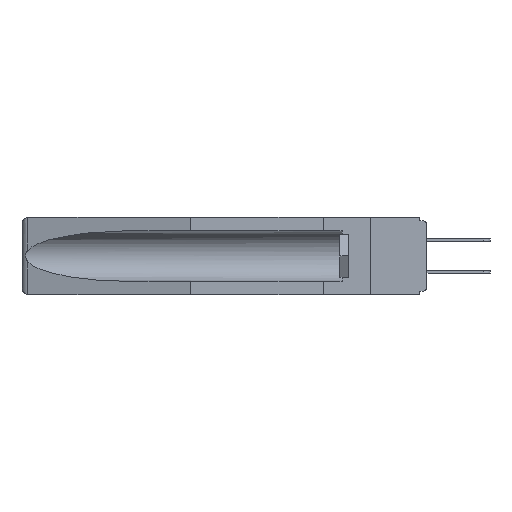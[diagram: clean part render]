
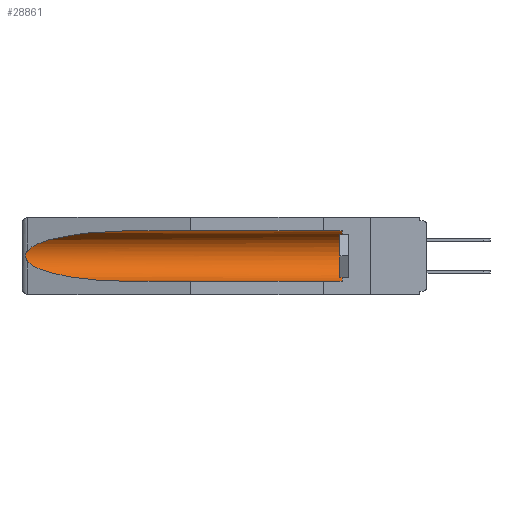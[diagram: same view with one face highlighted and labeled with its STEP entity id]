
A CAD part, left-side view. The second image highlights one B-rep face of the part: STEP entity #28861.
In plain terms, the highlighted cylindrical face has radius 2.857 mm (diameter 5.715 mm), a partial arc.
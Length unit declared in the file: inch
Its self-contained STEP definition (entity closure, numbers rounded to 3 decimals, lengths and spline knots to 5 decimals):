
#304 = CARTESIAN_POINT ( 'NONE',  ( 0.155, 1.07973, -0.284 ) ) ;
#995 = CARTESIAN_POINT ( 'NONE',  ( 0.26537, 1.52718, -0.19328 ) ) ;
#2540 = CARTESIAN_POINT ( 'NONE',  ( 0.26537, 1.52718, -0.19328 ) ) ;
#2613 = EDGE_CURVE ( 'NONE', #5798, #22632, #31333, .T. ) ;
#2690 = CARTESIAN_POINT ( 'NONE',  ( 0.155, -0.30754, -0.284 ) ) ;
#3827 = DIRECTION ( 'NONE',  ( 0., 1., 0. ) ) ;
#4141 = CARTESIAN_POINT ( 'NONE',  ( 0.155, 0.126, -0.284 ) ) ;
#4166 = EDGE_CURVE ( 'NONE', #13967, #22632, #28898, .T. ) ;
#4778 = CARTESIAN_POINT ( 'NONE',  ( 0.26654, 1.53092, -0.15636 ) ) ;
#5798 = VERTEX_POINT ( 'NONE', #4141 ) ;
#6088 = ORIENTED_EDGE ( 'NONE', *, *, #4166, .T. ) ;
#6415 = CYLINDRICAL_SURFACE ( 'NONE', #23253, 0.1125 ) ;
#6547 = CIRCLE ( 'NONE', #26962, 0.1125 ) ;
#7343 = CARTESIAN_POINT ( 'NONE',  ( 0.21114, 1.30732, -0.059 ) ) ;
#7671 = ORIENTED_EDGE ( 'NONE', *, *, #24232, .T. ) ;
#9757 = CARTESIAN_POINT ( 'NONE',  ( 0.2673, 1.53269, -0.17917 ) ) ;
#10486 = EDGE_CURVE ( 'NONE', #14201, #12692, #31477, .T. ) ;
#10596 = ORIENTED_EDGE ( 'NONE', *, *, #17280, .T. ) ;
#10952 = CARTESIAN_POINT ( 'NONE',  ( 0.155, 1.07973, -0.059 ) ) ;
#11768 = EDGE_CURVE ( 'NONE', #5798, #14201, #6547, .T. ) ;
#11940 = DIRECTION ( 'NONE',  ( 0., 1., 0. ) ) ;
#12079 = ORIENTED_EDGE ( 'NONE', *, *, #11768, .T. ) ;
#12133 = CARTESIAN_POINT ( 'NONE',  ( 0.2675, 1.53308, -0.17534 ) ) ;
#12256 = CARTESIAN_POINT ( 'NONE',  ( 0.2675, 1.53308, -0.16763 ) ) ;
#12260 = CARTESIAN_POINT ( 'NONE',  ( 0.21114, 1.30732, -0.284 ) ) ;
#12692 = VERTEX_POINT ( 'NONE', #10952 ) ;
#13586 = DIRECTION ( 'NONE',  ( 0., -1., 0. ) ) ;
#13647 = ORIENTED_EDGE ( 'NONE', *, *, #2613, .F. ) ;
#13967 = VERTEX_POINT ( 'NONE', #995 ) ;
#14201 = VERTEX_POINT ( 'NONE', #25459 ) ;
#14924 = CARTESIAN_POINT ( 'NONE',  ( 0.26537, 1.52718, -0.19328 ) ) ;
#15525 = CARTESIAN_POINT ( 'NONE',  ( 0.155, -0.30754, -0.1715 ) ) ;
#15832 = VECTOR ( 'NONE', #11940, 39.37008 ) ;
#15919 = CARTESIAN_POINT ( 'NONE',  ( 0.155, 0.126, -0.1715 ) ) ;
#16122 = DIRECTION ( 'NONE',  ( 0., 0., 1. ) ) ;
#16916 = CARTESIAN_POINT ( 'NONE',  ( 0.25451, 1.48313, -0.24835 ) ) ;
#17123 = CARTESIAN_POINT ( 'NONE',  ( 0.26597, 1.5296, -0.19026 ) ) ;
#17280 = EDGE_CURVE ( 'NONE', #12692, #18592, #25588, .T. ) ;
#18101 = ORIENTED_EDGE ( 'NONE', *, *, #10486, .T. ) ;
#18275 = FACE_OUTER_BOUND ( 'NONE', #19296, .T. ) ;
#18592 = VERTEX_POINT ( 'NONE', #21466 ) ;
#19296 = EDGE_LOOP ( 'NONE', ( #10596, #7671, #6088, #13647, #12079, #18101 ) ) ;
#20251 = VECTOR ( 'NONE', #22071, 39.37008 ) ;
#21466 = CARTESIAN_POINT ( 'NONE',  ( 0.26537, 1.52718, -0.14972 ) ) ;
#21719 = CARTESIAN_POINT ( 'NONE',  ( 0.2673, 1.5327, -0.16383 ) ) ;
#22071 = DIRECTION ( 'NONE',  ( 0., 1., 0. ) ) ;
#22632 = VERTEX_POINT ( 'NONE', #30739 ) ;
#22895 = DIRECTION ( 'NONE',  ( 0., 0., 1. ) ) ;
#23253 = AXIS2_PLACEMENT_3D ( 'NONE', #15525, #3827, #22895 ) ;
#24232 = EDGE_CURVE ( 'NONE', #18592, #13967, #29306, .T. ) ;
#24439 = CARTESIAN_POINT ( 'NONE',  ( 0.25451, 1.48313, -0.09465 ) ) ;
#25459 = CARTESIAN_POINT ( 'NONE',  ( 0.155, 0.126, -0.059 ) ) ;
#25588 =( BOUNDED_CURVE ( )  B_SPLINE_CURVE ( 3, ( #29211, #7343, #24439, #29330 ),
 .UNSPECIFIED., .F., .T. ) 
 B_SPLINE_CURVE_WITH_KNOTS ( ( 4, 4 ),
 ( 4.71239, 6.08839 ),
 .UNSPECIFIED. ) 
 CURVE ( )  GEOMETRIC_REPRESENTATION_ITEM ( )  RATIONAL_B_SPLINE_CURVE ( ( 1., 0.848, 0.848, 1. ) ) 
 REPRESENTATION_ITEM ( '' )  );
#26962 = AXIS2_PLACEMENT_3D ( 'NONE', #15919, #13586, #16122 ) ;
#28330 = CARTESIAN_POINT ( 'NONE',  ( 0.155, -0.30754, -0.059 ) ) ;
#28861 = ADVANCED_FACE ( 'NONE', ( #18275 ), #6415, .F. ) ;
#28898 =( BOUNDED_CURVE ( )  B_SPLINE_CURVE ( 3, ( #14924, #16916, #12260, #304 ),
 .UNSPECIFIED., .F., .F. ) 
 B_SPLINE_CURVE_WITH_KNOTS ( ( 4, 4 ),
 ( 0.1948, 1.5708 ),
 .UNSPECIFIED. ) 
 CURVE ( )  GEOMETRIC_REPRESENTATION_ITEM ( )  RATIONAL_B_SPLINE_CURVE ( ( 1., 0.848, 0.848, 1. ) ) 
 REPRESENTATION_ITEM ( '' )  );
#29175 = CARTESIAN_POINT ( 'NONE',  ( 0.26655, 1.53094, -0.18657 ) ) ;
#29211 = CARTESIAN_POINT ( 'NONE',  ( 0.155, 1.07973, -0.059 ) ) ;
#29289 = CARTESIAN_POINT ( 'NONE',  ( 0.26597, 1.52961, -0.15275 ) ) ;
#29306 = B_SPLINE_CURVE_WITH_KNOTS ( 'NONE', 3,
 ( #31447, #29289, #4778, #21719, #12256, #12133, #9757, #29175, #17123, #2540 ),
 .UNSPECIFIED., .F., .F.,
 ( 4, 2, 2, 2, 4 ),
 ( 0., 0.00029, 0.00058, 0.00087, 0.00117 ),
 .UNSPECIFIED. ) ;
#29330 = CARTESIAN_POINT ( 'NONE',  ( 0.26537, 1.52718, -0.14972 ) ) ;
#30739 = CARTESIAN_POINT ( 'NONE',  ( 0.155, 1.07973, -0.284 ) ) ;
#31333 = LINE ( 'NONE', #2690, #20251 ) ;
#31447 = CARTESIAN_POINT ( 'NONE',  ( 0.26537, 1.52718, -0.14972 ) ) ;
#31477 = LINE ( 'NONE', #28330, #15832 ) ;
